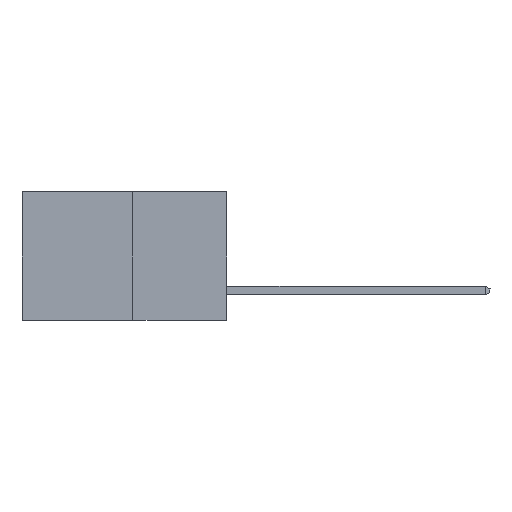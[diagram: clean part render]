
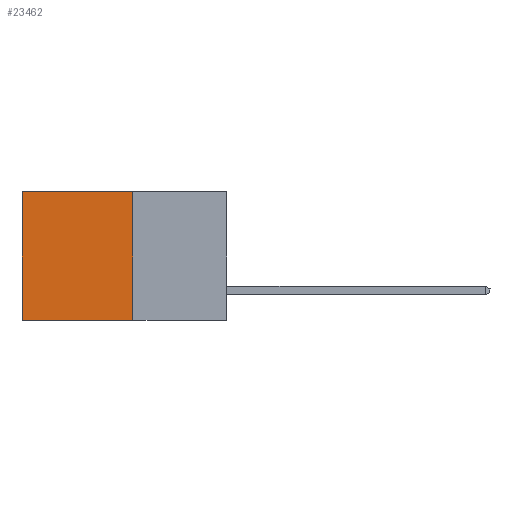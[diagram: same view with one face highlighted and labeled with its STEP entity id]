
A CAD part, left-side view. The second image highlights one B-rep face of the part: STEP entity #23462.
In plain terms, the highlighted planar face has unit normal (-1, 0, 0).
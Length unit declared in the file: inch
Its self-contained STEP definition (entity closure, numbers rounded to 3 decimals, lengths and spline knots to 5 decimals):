
#153 = DIRECTION ( 'NONE',  ( 0., 0., -1. ) ) ;
#603 = CARTESIAN_POINT ( 'NONE',  ( 0.277, 0.27, -0.37 ) ) ;
#1266 = DIRECTION ( 'NONE',  ( 0., 1., 0. ) ) ;
#2278 = DIRECTION ( 'NONE',  ( 0., 0., -1. ) ) ;
#4194 = EDGE_CURVE ( 'NONE', #14341, #16739, #28351, .T. ) ;
#5213 = DIRECTION ( 'NONE',  ( 0., 0., -1. ) ) ;
#5451 = ORIENTED_EDGE ( 'NONE', *, *, #5905, .T. ) ;
#5905 = EDGE_CURVE ( 'NONE', #16739, #27703, #19554, .T. ) ;
#6059 = CARTESIAN_POINT ( 'NONE',  ( 0.277, 0.27, 0. ) ) ;
#6680 = VECTOR ( 'NONE', #2278, 39.37008 ) ;
#6994 = ORIENTED_EDGE ( 'NONE', *, *, #21281, .F. ) ;
#9577 = VERTEX_POINT ( 'NONE', #23637 ) ;
#9737 = PLANE ( 'NONE',  #27030 ) ;
#10363 = DIRECTION ( 'NONE',  ( 0., 1., 0. ) ) ;
#10540 = CARTESIAN_POINT ( 'NONE',  ( 0.277, 0.27, 0. ) ) ;
#11390 = FACE_OUTER_BOUND ( 'NONE', #14951, .T. ) ;
#13282 = VECTOR ( 'NONE', #153, 39.37008 ) ;
#14341 = VERTEX_POINT ( 'NONE', #6059 ) ;
#14951 = EDGE_LOOP ( 'NONE', ( #5451, #22885, #6994, #20929 ) ) ;
#14991 = CARTESIAN_POINT ( 'NONE',  ( 0.277, 0.27, -0.37 ) ) ;
#16150 = LINE ( 'NONE', #16209, #13282 ) ;
#16209 = CARTESIAN_POINT ( 'NONE',  ( 0.277, 0.27, -0.37 ) ) ;
#16739 = VERTEX_POINT ( 'NONE', #21324 ) ;
#17405 = VECTOR ( 'NONE', #1266, 39.37008 ) ;
#18951 = DIRECTION ( 'NONE',  ( 1., 0., 0. ) ) ;
#19554 = LINE ( 'NONE', #22847, #6680 ) ;
#19656 = CARTESIAN_POINT ( 'NONE',  ( 0.277, 0.59, -0.37 ) ) ;
#20929 = ORIENTED_EDGE ( 'NONE', *, *, #4194, .T. ) ;
#21281 = EDGE_CURVE ( 'NONE', #14341, #9577, #16150, .T. ) ;
#21324 = CARTESIAN_POINT ( 'NONE',  ( 0.277, 0.59, 0. ) ) ;
#22452 = VECTOR ( 'NONE', #10363, 39.37008 ) ;
#22721 = LINE ( 'NONE', #14991, #17405 ) ;
#22847 = CARTESIAN_POINT ( 'NONE',  ( 0.277, 0.59, -0.37 ) ) ;
#22885 = ORIENTED_EDGE ( 'NONE', *, *, #29267, .F. ) ;
#23462 = ADVANCED_FACE ( 'NONE', ( #11390 ), #9737, .F. ) ;
#23637 = CARTESIAN_POINT ( 'NONE',  ( 0.277, 0.27, -0.37 ) ) ;
#27030 = AXIS2_PLACEMENT_3D ( 'NONE', #603, #18951, #5213 ) ;
#27703 = VERTEX_POINT ( 'NONE', #19656 ) ;
#28351 = LINE ( 'NONE', #10540, #22452 ) ;
#29267 = EDGE_CURVE ( 'NONE', #9577, #27703, #22721, .T. ) ;
